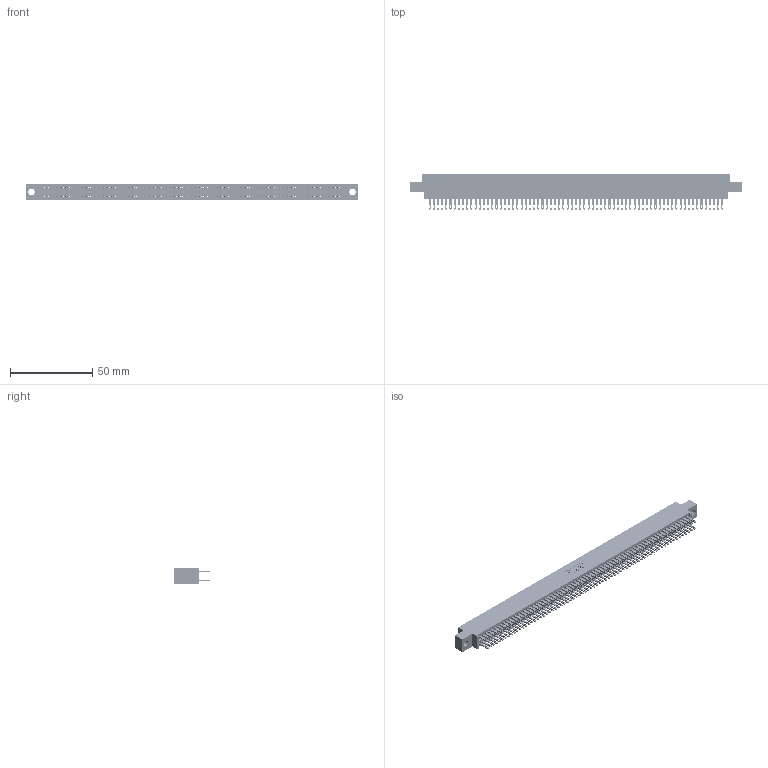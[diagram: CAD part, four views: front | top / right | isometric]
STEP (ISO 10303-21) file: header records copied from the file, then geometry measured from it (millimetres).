
FILE_DESCRIPTION (( 'STEP AP203' ), '1' );
FILE_NAME ('345-142-500-804.STEP', '2021-05-26T01:35:16', ( '' ), ( '' ), 'SwSTEP 2.0', 'SolidWorks 2020', '' );
FILE_SCHEMA (( 'CONFIG_CONTROL_DESIGN' ));
Length unit declared in the file: inch
Products named in the file (3): 345 Part_0.170 Offset - 0.156 Dia-TI; 345-292-001_345-293-100; 345-142-500-804
Assembly tree (143 placements, depth 2):
  345-142-500-804
    345 Part_0.170 Offset - 0.156 Dia-TI
    345-292-001_345-293-100  x142
Bounding box: 201.55 x 21.51 x 9.4 mm (x, y, z)
Volume: 20062.5 mm3; surface area: 31660.7 mm2
Topology: 143 solids, 143 shells, 6676 faces, 20411 edges, 13606 vertices
Faces by surface type: plane 3932, cylinder 2744
Entity records: 52285 total; most frequent: CARTESIAN_POINT 8742, ORIENTED_EDGE 8674, DIRECTION 7673, EDGE_CURVE 4337, LINE 3917, VECTOR 3917, VERTEX_POINT 2890, AXIS2_PLACEMENT_3D 1878
